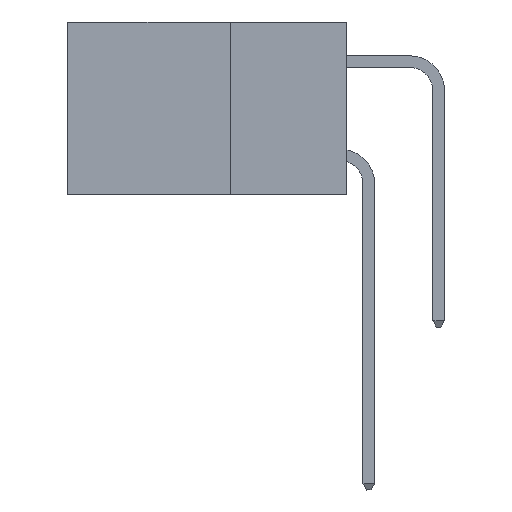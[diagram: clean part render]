
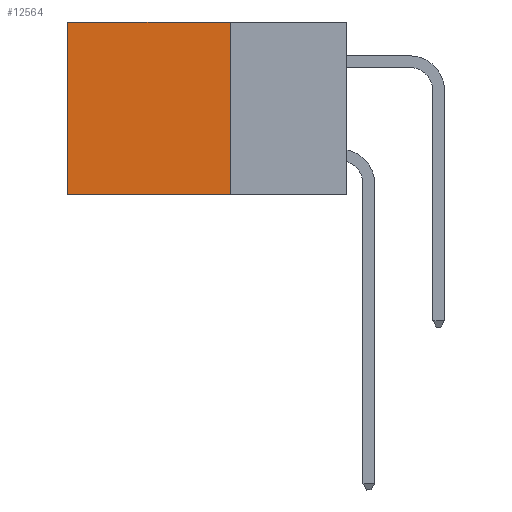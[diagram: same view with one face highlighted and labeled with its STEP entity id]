
A CAD part, left-side view. The second image highlights one B-rep face of the part: STEP entity #12564.
In plain terms, the highlighted planar face has unit normal (-1, 0, 0).
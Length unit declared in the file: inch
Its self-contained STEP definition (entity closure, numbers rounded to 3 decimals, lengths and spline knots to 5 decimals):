
#640 = VERTEX_POINT ( 'NONE', #7683 ) ;
#729 = CARTESIAN_POINT ( 'NONE',  ( 0.2875, 0.25, 0. ) ) ;
#848 = VERTEX_POINT ( 'NONE', #12636 ) ;
#1381 = FACE_OUTER_BOUND ( 'NONE', #3014, .T. ) ;
#1631 = DIRECTION ( 'NONE',  ( 0., 1., 0. ) ) ;
#1757 = ORIENTED_EDGE ( 'NONE', *, *, #14527, .F. ) ;
#2050 = AXIS2_PLACEMENT_3D ( 'NONE', #729, #14790, #5331 ) ;
#2516 = CARTESIAN_POINT ( 'NONE',  ( 0.2875, 0.25, 0. ) ) ;
#2842 = CARTESIAN_POINT ( 'NONE',  ( 0.2875, 0.25, 0. ) ) ;
#3014 = EDGE_LOOP ( 'NONE', ( #12827, #8838, #1757, #11986 ) ) ;
#4209 = VECTOR ( 'NONE', #6231, 39.37008 ) ;
#4432 = VERTEX_POINT ( 'NONE', #2842 ) ;
#4461 = VECTOR ( 'NONE', #6303, 39.37008 ) ;
#5301 = EDGE_CURVE ( 'NONE', #4432, #12556, #5866, .T. ) ;
#5331 = DIRECTION ( 'NONE',  ( 0., 0., -1. ) ) ;
#5866 = LINE ( 'NONE', #2516, #4209 ) ;
#6117 = LINE ( 'NONE', #13389, #14109 ) ;
#6231 = DIRECTION ( 'NONE',  ( 0., 1., 0. ) ) ;
#6303 = DIRECTION ( 'NONE',  ( 0., 0., -1. ) ) ;
#6482 = LINE ( 'NONE', #13375, #4461 ) ;
#7158 = EDGE_CURVE ( 'NONE', #640, #848, #6117, .T. ) ;
#7683 = CARTESIAN_POINT ( 'NONE',  ( 0.2875, 0.25, -0.37 ) ) ;
#7751 = CARTESIAN_POINT ( 'NONE',  ( 0.2875, 0.6, 0. ) ) ;
#8838 = ORIENTED_EDGE ( 'NONE', *, *, #7158, .F. ) ;
#8925 = EDGE_CURVE ( 'NONE', #12556, #848, #11000, .T. ) ;
#9144 = CARTESIAN_POINT ( 'NONE',  ( 0.2875, 0.6, 0. ) ) ;
#9342 = VECTOR ( 'NONE', #10521, 39.37008 ) ;
#10521 = DIRECTION ( 'NONE',  ( 0., 0., -1. ) ) ;
#11000 = LINE ( 'NONE', #9144, #9342 ) ;
#11986 = ORIENTED_EDGE ( 'NONE', *, *, #5301, .T. ) ;
#12556 = VERTEX_POINT ( 'NONE', #7751 ) ;
#12564 = ADVANCED_FACE ( 'NONE', ( #1381 ), #13541, .F. ) ;
#12636 = CARTESIAN_POINT ( 'NONE',  ( 0.2875, 0.6, -0.37 ) ) ;
#12827 = ORIENTED_EDGE ( 'NONE', *, *, #8925, .T. ) ;
#13375 = CARTESIAN_POINT ( 'NONE',  ( 0.2875, 0.25, 0. ) ) ;
#13389 = CARTESIAN_POINT ( 'NONE',  ( 0.2875, 0.25, -0.37 ) ) ;
#13541 = PLANE ( 'NONE',  #2050 ) ;
#14109 = VECTOR ( 'NONE', #1631, 39.37008 ) ;
#14527 = EDGE_CURVE ( 'NONE', #4432, #640, #6482, .T. ) ;
#14790 = DIRECTION ( 'NONE',  ( 1., 0., 0. ) ) ;
